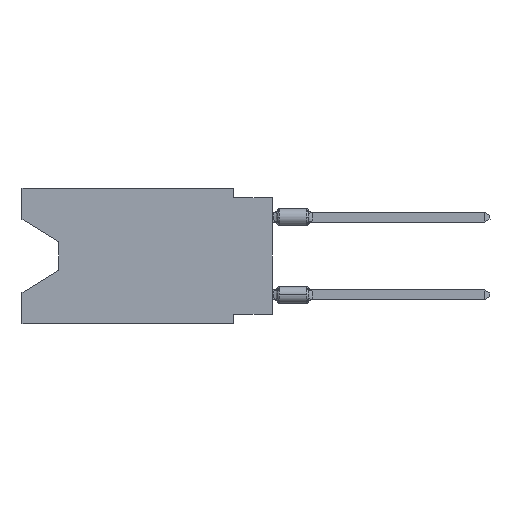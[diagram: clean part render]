
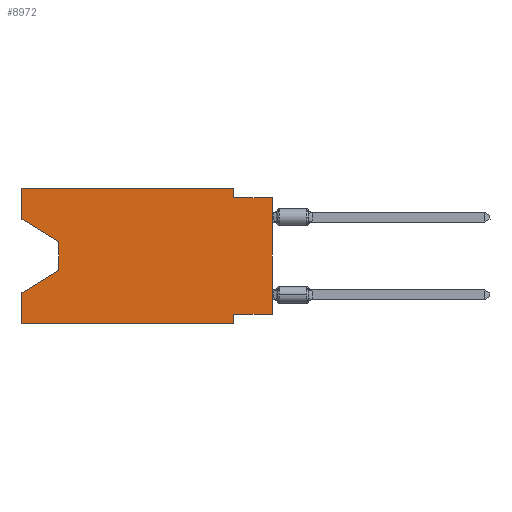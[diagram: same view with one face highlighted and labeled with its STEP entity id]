
A CAD part, left-side view. The second image highlights one B-rep face of the part: STEP entity #8972.
In plain terms, the highlighted planar face has unit normal (-1, 0, 0).
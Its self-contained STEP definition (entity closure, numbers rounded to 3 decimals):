
#282 = LINE ( 'NONE', #4312, #9018 ) ;
#368 = ORIENTED_EDGE ( 'NONE', *, *, #26692, .T. ) ;
#883 = VECTOR ( 'NONE', #15521, 1000. ) ;
#886 = VERTEX_POINT ( 'NONE', #8499 ) ;
#1834 = EDGE_CURVE ( 'NONE', #4618, #16769, #13806, .T. ) ;
#1869 = EDGE_CURVE ( 'NONE', #886, #16769, #10032, .T. ) ;
#2041 = VECTOR ( 'NONE', #26045, 1000. ) ;
#2129 = VERTEX_POINT ( 'NONE', #2234 ) ;
#2234 = CARTESIAN_POINT ( 'NONE',  ( 0., 2.54, -8.255 ) ) ;
#2900 = VERTEX_POINT ( 'NONE', #12744 ) ;
#3412 = CARTESIAN_POINT ( 'NONE',  ( 0., 2.54, 0. ) ) ;
#3446 = DIRECTION ( 'NONE',  ( 0., 0., 1. ) ) ;
#3709 = CARTESIAN_POINT ( 'NONE',  ( 0., 16.383, 0. ) ) ;
#3851 = VECTOR ( 'NONE', #10356, 1000. ) ;
#4312 = CARTESIAN_POINT ( 'NONE',  ( 0., 13.97, -3.505 ) ) ;
#4616 = EDGE_CURVE ( 'NONE', #11426, #4618, #26312, .T. ) ;
#4618 = VERTEX_POINT ( 'NONE', #23683 ) ;
#4697 = AXIS2_PLACEMENT_3D ( 'NONE', #15531, #15389, #9134 ) ;
#4757 = ORIENTED_EDGE ( 'NONE', *, *, #16471, .T. ) ;
#4879 = EDGE_CURVE ( 'NONE', #2129, #11045, #27134, .T. ) ;
#4880 = CARTESIAN_POINT ( 'NONE',  ( 0., 13.97, -5.385 ) ) ;
#5135 = VECTOR ( 'NONE', #27220, 1000. ) ;
#5296 = LINE ( 'NONE', #4880, #7649 ) ;
#5536 = LINE ( 'NONE', #3709, #12138 ) ;
#6301 = EDGE_CURVE ( 'NONE', #8075, #23847, #23938, .T. ) ;
#6778 = FACE_OUTER_BOUND ( 'NONE', #11182, .T. ) ;
#6875 = ORIENTED_EDGE ( 'NONE', *, *, #26218, .F. ) ;
#7633 = ORIENTED_EDGE ( 'NONE', *, *, #16092, .T. ) ;
#7649 = VECTOR ( 'NONE', #13374, 1000. ) ;
#8075 = VERTEX_POINT ( 'NONE', #14505 ) ;
#8414 = VERTEX_POINT ( 'NONE', #16952 ) ;
#8499 = CARTESIAN_POINT ( 'NONE',  ( 0., 0., -8.255 ) ) ;
#8972 = ADVANCED_FACE ( 'NONE', ( #6778 ), #21626, .F. ) ;
#8991 = LINE ( 'NONE', #25641, #883 ) ;
#9018 = VECTOR ( 'NONE', #23193, 1000. ) ;
#9134 = DIRECTION ( 'NONE',  ( 0., 0., -1. ) ) ;
#9804 = CARTESIAN_POINT ( 'NONE',  ( 0., 13.97, -5.385 ) ) ;
#10032 = LINE ( 'NONE', #18901, #5135 ) ;
#10356 = DIRECTION ( 'NONE',  ( 0., 0., -1. ) ) ;
#10860 = CARTESIAN_POINT ( 'NONE',  ( 0., 0., -0.635 ) ) ;
#11045 = VERTEX_POINT ( 'NONE', #17780 ) ;
#11182 = EDGE_LOOP ( 'NONE', ( #7633, #368, #21074, #18439, #4757, #21175, #16052, #25302, #15844, #26195, #22352, #6875 ) ) ;
#11426 = VERTEX_POINT ( 'NONE', #3412 ) ;
#11615 = CARTESIAN_POINT ( 'NONE',  ( 0., 16.383, -2.038 ) ) ;
#11707 = CARTESIAN_POINT ( 'NONE',  ( 0., 0., -0.635 ) ) ;
#12138 = VECTOR ( 'NONE', #3446, 1000. ) ;
#12175 = VECTOR ( 'NONE', #21706, 1000. ) ;
#12581 = CARTESIAN_POINT ( 'NONE',  ( 0., 2.54, -8.89 ) ) ;
#12744 = CARTESIAN_POINT ( 'NONE',  ( 0., 13.97, -3.505 ) ) ;
#13374 = DIRECTION ( 'NONE',  ( 0., 0.855, -0.519 ) ) ;
#13806 = LINE ( 'NONE', #11707, #20653 ) ;
#14505 = CARTESIAN_POINT ( 'NONE',  ( 0., 16.383, -8.89 ) ) ;
#15212 = DIRECTION ( 'NONE',  ( 0., 0., 1. ) ) ;
#15267 = VERTEX_POINT ( 'NONE', #23780 ) ;
#15317 = EDGE_CURVE ( 'NONE', #886, #2129, #22114, .T. ) ;
#15389 = DIRECTION ( 'NONE',  ( 1., 0., 0. ) ) ;
#15521 = DIRECTION ( 'NONE',  ( 0., -1., 0. ) ) ;
#15531 = CARTESIAN_POINT ( 'NONE',  ( 0., 16.383, 0. ) ) ;
#15616 = CARTESIAN_POINT ( 'NONE',  ( 0., 16.383, -8.89 ) ) ;
#15844 = ORIENTED_EDGE ( 'NONE', *, *, #1834, .F. ) ;
#16052 = ORIENTED_EDGE ( 'NONE', *, *, #15317, .F. ) ;
#16092 = EDGE_CURVE ( 'NONE', #8414, #2900, #19940, .T. ) ;
#16471 = EDGE_CURVE ( 'NONE', #8075, #11045, #22255, .T. ) ;
#16769 = VERTEX_POINT ( 'NONE', #10860 ) ;
#16952 = CARTESIAN_POINT ( 'NONE',  ( 0., 16.383, -2.038 ) ) ;
#17446 = CARTESIAN_POINT ( 'NONE',  ( 0., 2.54, 0. ) ) ;
#17692 = DIRECTION ( 'NONE',  ( 0., -1., 0. ) ) ;
#17699 = CARTESIAN_POINT ( 'NONE',  ( 0., 16.383, 0. ) ) ;
#17780 = CARTESIAN_POINT ( 'NONE',  ( 0., 2.54, -8.89 ) ) ;
#18439 = ORIENTED_EDGE ( 'NONE', *, *, #6301, .F. ) ;
#18901 = CARTESIAN_POINT ( 'NONE',  ( 0., 0., 0. ) ) ;
#19940 = LINE ( 'NONE', #11615, #23725 ) ;
#20167 = DIRECTION ( 'NONE',  ( 0., -1., 0. ) ) ;
#20593 = VERTEX_POINT ( 'NONE', #9804 ) ;
#20653 = VECTOR ( 'NONE', #20167, 1000. ) ;
#21074 = ORIENTED_EDGE ( 'NONE', *, *, #24419, .T. ) ;
#21082 = VECTOR ( 'NONE', #17692, 1000. ) ;
#21140 = VECTOR ( 'NONE', #15212, 1000. ) ;
#21175 = ORIENTED_EDGE ( 'NONE', *, *, #4879, .F. ) ;
#21571 = CARTESIAN_POINT ( 'NONE',  ( 0., 0., -8.255 ) ) ;
#21626 = PLANE ( 'NONE',  #4697 ) ;
#21706 = DIRECTION ( 'NONE',  ( 0., 1., 0. ) ) ;
#21716 = CARTESIAN_POINT ( 'NONE',  ( 0., 16.383, -6.852 ) ) ;
#22114 = LINE ( 'NONE', #21571, #12175 ) ;
#22179 = EDGE_CURVE ( 'NONE', #15267, #11426, #8991, .T. ) ;
#22255 = LINE ( 'NONE', #15616, #21082 ) ;
#22352 = ORIENTED_EDGE ( 'NONE', *, *, #22179, .F. ) ;
#23193 = DIRECTION ( 'NONE',  ( 0., 0., -1. ) ) ;
#23683 = CARTESIAN_POINT ( 'NONE',  ( 0., 2.54, -0.635 ) ) ;
#23725 = VECTOR ( 'NONE', #26177, 1000. ) ;
#23780 = CARTESIAN_POINT ( 'NONE',  ( 0., 16.383, 0. ) ) ;
#23847 = VERTEX_POINT ( 'NONE', #21716 ) ;
#23938 = LINE ( 'NONE', #17699, #21140 ) ;
#24419 = EDGE_CURVE ( 'NONE', #20593, #23847, #5296, .T. ) ;
#25302 = ORIENTED_EDGE ( 'NONE', *, *, #1869, .T. ) ;
#25641 = CARTESIAN_POINT ( 'NONE',  ( 0., 16.383, 0. ) ) ;
#26045 = DIRECTION ( 'NONE',  ( 0., 0., -1. ) ) ;
#26177 = DIRECTION ( 'NONE',  ( 0., -0.855, -0.519 ) ) ;
#26195 = ORIENTED_EDGE ( 'NONE', *, *, #4616, .F. ) ;
#26218 = EDGE_CURVE ( 'NONE', #8414, #15267, #5536, .T. ) ;
#26312 = LINE ( 'NONE', #17446, #2041 ) ;
#26692 = EDGE_CURVE ( 'NONE', #2900, #20593, #282, .T. ) ;
#27134 = LINE ( 'NONE', #12581, #3851 ) ;
#27220 = DIRECTION ( 'NONE',  ( 0., 0., 1. ) ) ;
